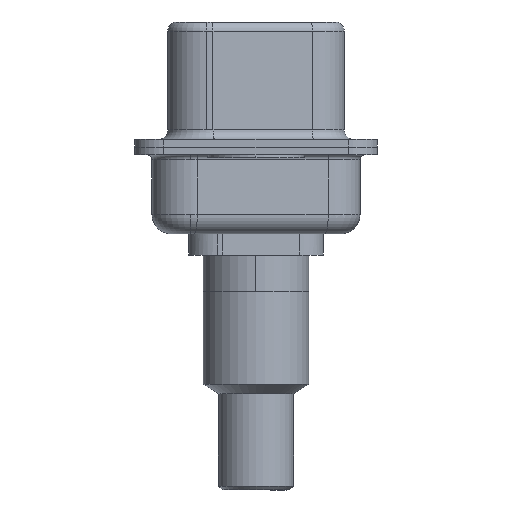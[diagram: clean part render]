
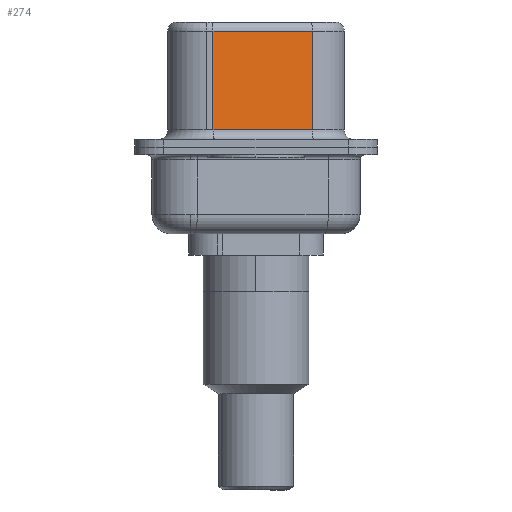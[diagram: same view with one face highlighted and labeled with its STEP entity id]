
A CAD part, left-side view. The second image highlights one B-rep face of the part: STEP entity #274.
In plain terms, the highlighted planar face has unit normal (-0.985, -0.174, 0).
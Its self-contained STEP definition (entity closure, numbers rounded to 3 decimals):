
#212 = LINE ( 'NONE', #11704, #700 ) ;
#274 = ADVANCED_FACE ( 'NONE', ( #16514 ), #5647, .F. ) ;
#634 = LINE ( 'NONE', #12770, #8283 ) ;
#700 = VECTOR ( 'NONE', #12500, 1000. ) ;
#938 = DIRECTION ( 'NONE',  ( -0.174, 0.985, 0. ) ) ;
#1723 = CARTESIAN_POINT ( 'NONE',  ( 3.655, 2.233, 6.52 ) ) ;
#2051 = EDGE_CURVE ( 'NONE', #8413, #9415, #212, .T. ) ;
#2335 = VECTOR ( 'NONE', #15169, 1000. ) ;
#2345 = ORIENTED_EDGE ( 'NONE', *, *, #2051, .T. ) ;
#2785 = LINE ( 'NONE', #1723, #2335 ) ;
#3562 = ORIENTED_EDGE ( 'NONE', *, *, #12680, .T. ) ;
#3884 = LINE ( 'NONE', #15710, #14965 ) ;
#5647 = PLANE ( 'NONE',  #9398 ) ;
#5656 = VERTEX_POINT ( 'NONE', #10249 ) ;
#6735 = VERTEX_POINT ( 'NONE', #15909 ) ;
#6967 = CARTESIAN_POINT ( 'NONE',  ( 3.655, 2.233, 0.9 ) ) ;
#7086 = CARTESIAN_POINT ( 'NONE',  ( 4.565, -2.927, 0.9 ) ) ;
#7325 = EDGE_CURVE ( 'NONE', #6735, #8413, #2785, .T. ) ;
#8032 = ORIENTED_EDGE ( 'NONE', *, *, #7325, .T. ) ;
#8283 = VECTOR ( 'NONE', #938, 1000. ) ;
#8413 = VERTEX_POINT ( 'NONE', #6967 ) ;
#9398 = AXIS2_PLACEMENT_3D ( 'NONE', #12527, #12651, #12774 ) ;
#9415 = VERTEX_POINT ( 'NONE', #7086 ) ;
#10249 = CARTESIAN_POINT ( 'NONE',  ( 4.565, -2.927, 6.02 ) ) ;
#10449 = EDGE_CURVE ( 'NONE', #5656, #9415, #3884, .T. ) ;
#11704 = CARTESIAN_POINT ( 'NONE',  ( 4.565, -2.927, 0.9 ) ) ;
#12500 = DIRECTION ( 'NONE',  ( 0.174, -0.985, 0. ) ) ;
#12527 = CARTESIAN_POINT ( 'NONE',  ( 4.565, -2.927, 6.52 ) ) ;
#12651 = DIRECTION ( 'NONE',  ( 0.985, 0.174, 0. ) ) ;
#12680 = EDGE_CURVE ( 'NONE', #5656, #6735, #634, .T. ) ;
#12770 = CARTESIAN_POINT ( 'NONE',  ( 4.565, -2.927, 6.02 ) ) ;
#12774 = DIRECTION ( 'NONE',  ( -0.174, 0.985, 0. ) ) ;
#13567 = ORIENTED_EDGE ( 'NONE', *, *, #10449, .F. ) ;
#14418 = DIRECTION ( 'NONE',  ( 0., 0., -1. ) ) ;
#14965 = VECTOR ( 'NONE', #14418, 1000. ) ;
#15169 = DIRECTION ( 'NONE',  ( 0., 0., -1. ) ) ;
#15710 = CARTESIAN_POINT ( 'NONE',  ( 4.565, -2.927, 6.52 ) ) ;
#15909 = CARTESIAN_POINT ( 'NONE',  ( 3.655, 2.233, 6.02 ) ) ;
#16514 = FACE_OUTER_BOUND ( 'NONE', #17021, .T. ) ;
#17021 = EDGE_LOOP ( 'NONE', ( #13567, #3562, #8032, #2345 ) ) ;
